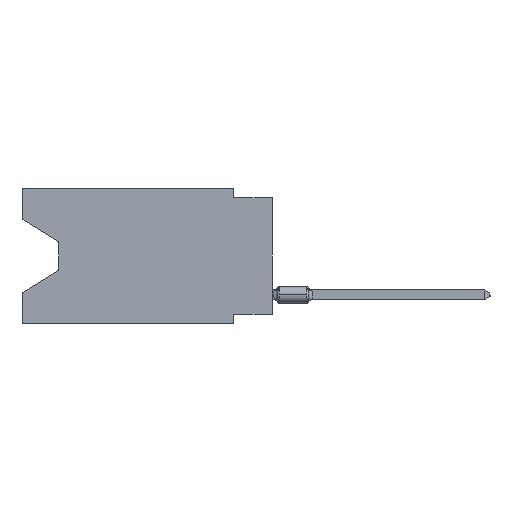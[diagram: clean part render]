
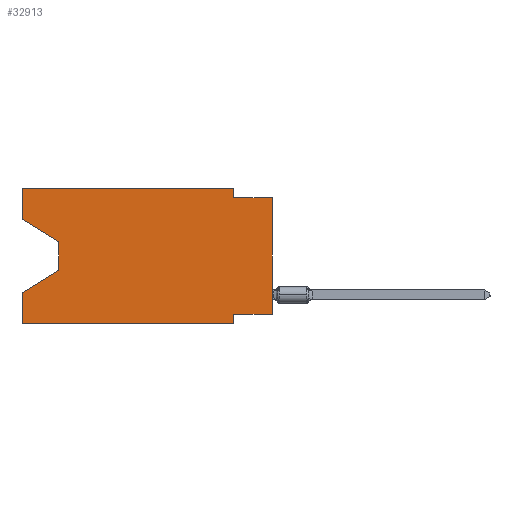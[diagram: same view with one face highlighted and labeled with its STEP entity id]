
A CAD part, left-side view. The second image highlights one B-rep face of the part: STEP entity #32913.
In plain terms, the highlighted planar face has unit normal (-1, 0, 0).
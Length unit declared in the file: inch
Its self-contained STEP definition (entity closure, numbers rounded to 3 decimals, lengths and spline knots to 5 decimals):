
#71 = CARTESIAN_POINT ( 'NONE',  ( 0., 0.645, -0.26975 ) ) ;
#222 = ORIENTED_EDGE ( 'NONE', *, *, #18816, .F. ) ;
#883 = CARTESIAN_POINT ( 'NONE',  ( 0., 0.55, -0.138 ) ) ;
#2234 = DIRECTION ( 'NONE',  ( 0., 0., -1. ) ) ;
#2573 = CARTESIAN_POINT ( 'NONE',  ( 0., 0., -0.025 ) ) ;
#3334 = EDGE_CURVE ( 'NONE', #36867, #19364, #35027, .T. ) ;
#3374 = EDGE_CURVE ( 'NONE', #36963, #25277, #34832, .T. ) ;
#4070 = CARTESIAN_POINT ( 'NONE',  ( 0., 0.55, -0.212 ) ) ;
#4132 = VECTOR ( 'NONE', #28333, 39.37008 ) ;
#4233 = VECTOR ( 'NONE', #32582, 39.37008 ) ;
#4289 = AXIS2_PLACEMENT_3D ( 'NONE', #11335, #8244, #10767 ) ;
#4362 = VECTOR ( 'NONE', #2234, 39.37008 ) ;
#4449 = DIRECTION ( 'NONE',  ( 0., 1., 0. ) ) ;
#4632 = ORIENTED_EDGE ( 'NONE', *, *, #24514, .T. ) ;
#5098 = CARTESIAN_POINT ( 'NONE',  ( 0., 0.1, -0.025 ) ) ;
#5472 = ORIENTED_EDGE ( 'NONE', *, *, #23576, .T. ) ;
#6718 = VECTOR ( 'NONE', #27611, 39.37008 ) ;
#6999 = EDGE_LOOP ( 'NONE', ( #21580, #8743, #20658, #222, #4632, #38186, #18601, #5472, #30153, #33978, #20230, #28704 ) ) ;
#7257 = CARTESIAN_POINT ( 'NONE',  ( 0., 0.55, -0.138 ) ) ;
#7591 = DIRECTION ( 'NONE',  ( 0., 0., 1. ) ) ;
#8153 = DIRECTION ( 'NONE',  ( 0., 0., -1. ) ) ;
#8244 = DIRECTION ( 'NONE',  ( 1., 0., 0. ) ) ;
#8376 = VECTOR ( 'NONE', #11623, 39.37008 ) ;
#8743 = ORIENTED_EDGE ( 'NONE', *, *, #16749, .T. ) ;
#9216 = VERTEX_POINT ( 'NONE', #71 ) ;
#10767 = DIRECTION ( 'NONE',  ( 0., 0., -1. ) ) ;
#11335 = CARTESIAN_POINT ( 'NONE',  ( 0., 0.645, 0. ) ) ;
#11623 = DIRECTION ( 'NONE',  ( 0., -1., 0. ) ) ;
#12137 = VECTOR ( 'NONE', #14784, 39.37008 ) ;
#12896 = EDGE_CURVE ( 'NONE', #19364, #36607, #22364, .T. ) ;
#13320 = VECTOR ( 'NONE', #8153, 39.37008 ) ;
#13655 = LINE ( 'NONE', #34141, #4132 ) ;
#14019 = VERTEX_POINT ( 'NONE', #16953 ) ;
#14414 = VERTEX_POINT ( 'NONE', #28505 ) ;
#14755 = LINE ( 'NONE', #2573, #21060 ) ;
#14784 = DIRECTION ( 'NONE',  ( 0., 0., 1. ) ) ;
#15825 = CARTESIAN_POINT ( 'NONE',  ( 0., 0.645, 0. ) ) ;
#15923 = VECTOR ( 'NONE', #28328, 39.37008 ) ;
#16067 = CARTESIAN_POINT ( 'NONE',  ( 0., 0., -0.325 ) ) ;
#16071 = LINE ( 'NONE', #4070, #4233 ) ;
#16749 = EDGE_CURVE ( 'NONE', #35235, #14414, #27937, .T. ) ;
#16953 = CARTESIAN_POINT ( 'NONE',  ( 0., 0., -0.325 ) ) ;
#18601 = ORIENTED_EDGE ( 'NONE', *, *, #20459, .F. ) ;
#18816 = EDGE_CURVE ( 'NONE', #28327, #9216, #30983, .T. ) ;
#19138 = VECTOR ( 'NONE', #4449, 39.37008 ) ;
#19153 = EDGE_CURVE ( 'NONE', #19602, #36867, #33416, .T. ) ;
#19184 = CARTESIAN_POINT ( 'NONE',  ( 0., 0.645, 0. ) ) ;
#19199 = CARTESIAN_POINT ( 'NONE',  ( 0., 0.645, -0.35 ) ) ;
#19364 = VERTEX_POINT ( 'NONE', #32628 ) ;
#19602 = VERTEX_POINT ( 'NONE', #30455 ) ;
#19855 = PLANE ( 'NONE',  #4289 ) ;
#20230 = ORIENTED_EDGE ( 'NONE', *, *, #3334, .F. ) ;
#20325 = CARTESIAN_POINT ( 'NONE',  ( 0., 0.1, -0.325 ) ) ;
#20459 = EDGE_CURVE ( 'NONE', #14019, #36963, #33661, .T. ) ;
#20658 = ORIENTED_EDGE ( 'NONE', *, *, #29910, .T. ) ;
#21060 = VECTOR ( 'NONE', #21253, 39.37008 ) ;
#21253 = DIRECTION ( 'NONE',  ( 0., -1., 0. ) ) ;
#21580 = ORIENTED_EDGE ( 'NONE', *, *, #28150, .T. ) ;
#22364 = LINE ( 'NONE', #34721, #4362 ) ;
#22860 = CARTESIAN_POINT ( 'NONE',  ( 0., 0.1, -0.35 ) ) ;
#23244 = CARTESIAN_POINT ( 'NONE',  ( 0., 0.645, 0. ) ) ;
#23576 = EDGE_CURVE ( 'NONE', #14019, #35025, #38187, .T. ) ;
#24250 = CARTESIAN_POINT ( 'NONE',  ( 0., 0., 0. ) ) ;
#24514 = EDGE_CURVE ( 'NONE', #28327, #25277, #27700, .T. ) ;
#25277 = VERTEX_POINT ( 'NONE', #30653 ) ;
#27314 = DIRECTION ( 'NONE',  ( 0., -1., 0. ) ) ;
#27611 = DIRECTION ( 'NONE',  ( 0., 0., 1. ) ) ;
#27700 = LINE ( 'NONE', #19199, #34941 ) ;
#27937 = LINE ( 'NONE', #7257, #15923 ) ;
#28150 = EDGE_CURVE ( 'NONE', #19602, #35235, #13655, .T. ) ;
#28327 = VERTEX_POINT ( 'NONE', #33030 ) ;
#28328 = DIRECTION ( 'NONE',  ( 0., 0., -1. ) ) ;
#28333 = DIRECTION ( 'NONE',  ( 0., -0.855, -0.519 ) ) ;
#28505 = CARTESIAN_POINT ( 'NONE',  ( 0., 0.55, -0.212 ) ) ;
#28704 = ORIENTED_EDGE ( 'NONE', *, *, #19153, .F. ) ;
#29910 = EDGE_CURVE ( 'NONE', #14414, #9216, #16071, .T. ) ;
#30153 = ORIENTED_EDGE ( 'NONE', *, *, #34275, .F. ) ;
#30455 = CARTESIAN_POINT ( 'NONE',  ( 0., 0.645, -0.08025 ) ) ;
#30653 = CARTESIAN_POINT ( 'NONE',  ( 0., 0.1, -0.35 ) ) ;
#30983 = LINE ( 'NONE', #31898, #32048 ) ;
#31898 = CARTESIAN_POINT ( 'NONE',  ( 0., 0.645, 0. ) ) ;
#32048 = VECTOR ( 'NONE', #7591, 39.37008 ) ;
#32582 = DIRECTION ( 'NONE',  ( 0., 0.855, -0.519 ) ) ;
#32628 = CARTESIAN_POINT ( 'NONE',  ( 0., 0.1, 0. ) ) ;
#32913 = ADVANCED_FACE ( 'NONE', ( #38023 ), #19855, .F. ) ;
#33001 = CARTESIAN_POINT ( 'NONE',  ( 0., 0., -0.025 ) ) ;
#33030 = CARTESIAN_POINT ( 'NONE',  ( 0., 0.645, -0.35 ) ) ;
#33416 = LINE ( 'NONE', #15825, #6718 ) ;
#33661 = LINE ( 'NONE', #16067, #19138 ) ;
#33978 = ORIENTED_EDGE ( 'NONE', *, *, #12896, .F. ) ;
#34141 = CARTESIAN_POINT ( 'NONE',  ( 0., 0.645, -0.08025 ) ) ;
#34275 = EDGE_CURVE ( 'NONE', #36607, #35025, #14755, .T. ) ;
#34721 = CARTESIAN_POINT ( 'NONE',  ( 0., 0.1, 0. ) ) ;
#34832 = LINE ( 'NONE', #22860, #13320 ) ;
#34941 = VECTOR ( 'NONE', #27314, 39.37008 ) ;
#35025 = VERTEX_POINT ( 'NONE', #33001 ) ;
#35027 = LINE ( 'NONE', #23244, #8376 ) ;
#35235 = VERTEX_POINT ( 'NONE', #883 ) ;
#36607 = VERTEX_POINT ( 'NONE', #5098 ) ;
#36867 = VERTEX_POINT ( 'NONE', #19184 ) ;
#36963 = VERTEX_POINT ( 'NONE', #20325 ) ;
#38023 = FACE_OUTER_BOUND ( 'NONE', #6999, .T. ) ;
#38186 = ORIENTED_EDGE ( 'NONE', *, *, #3374, .F. ) ;
#38187 = LINE ( 'NONE', #24250, #12137 ) ;
